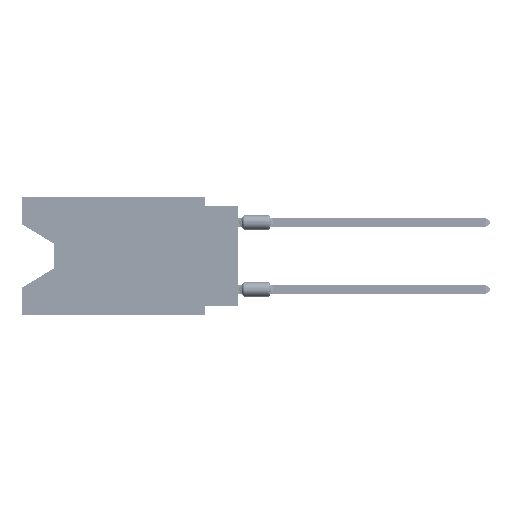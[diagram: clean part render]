
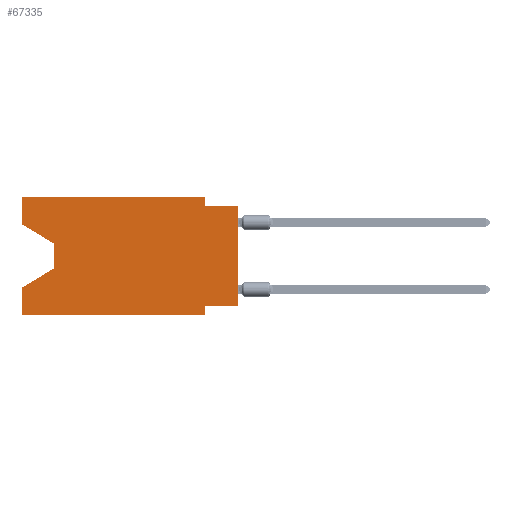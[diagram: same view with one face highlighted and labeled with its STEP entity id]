
A CAD part, left-side view. The second image highlights one B-rep face of the part: STEP entity #67335.
In plain terms, the highlighted planar face has unit normal (-1, 0, 0).
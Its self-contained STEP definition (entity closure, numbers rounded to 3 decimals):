
#154 = VERTEX_POINT ( 'NONE', #52740 ) ;
#1764 = EDGE_CURVE ( 'NONE', #3936, #50793, #80756, .T. ) ;
#3936 = VERTEX_POINT ( 'NONE', #56973 ) ;
#4220 = ORIENTED_EDGE ( 'NONE', *, *, #75615, .F. ) ;
#5803 = VECTOR ( 'NONE', #24884, 1000. ) ;
#6697 = PLANE ( 'NONE',  #82722 ) ;
#6852 = DIRECTION ( 'NONE',  ( 0., 0., -1. ) ) ;
#13258 = FACE_OUTER_BOUND ( 'NONE', #33063, .T. ) ;
#13718 = CARTESIAN_POINT ( 'NONE',  ( 0., 2.54, 0. ) ) ;
#14518 = DIRECTION ( 'NONE',  ( 0., 0., -1. ) ) ;
#15775 = DIRECTION ( 'NONE',  ( 0., -0.855, -0.519 ) ) ;
#16699 = CARTESIAN_POINT ( 'NONE',  ( 0., 16.383, 0. ) ) ;
#16708 = CARTESIAN_POINT ( 'NONE',  ( 0., 13.97, -5.385 ) ) ;
#16961 = ORIENTED_EDGE ( 'NONE', *, *, #58925, .F. ) ;
#18327 = LINE ( 'NONE', #37089, #5803 ) ;
#19431 = ORIENTED_EDGE ( 'NONE', *, *, #78847, .F. ) ;
#19486 = DIRECTION ( 'NONE',  ( 0., 0., 1. ) ) ;
#20074 = LINE ( 'NONE', #40119, #56451 ) ;
#20825 = CARTESIAN_POINT ( 'NONE',  ( 0., 16.383, 0. ) ) ;
#21880 = CARTESIAN_POINT ( 'NONE',  ( 0., 2.54, -8.89 ) ) ;
#22563 = CARTESIAN_POINT ( 'NONE',  ( 0., 16.383, -8.89 ) ) ;
#24884 = DIRECTION ( 'NONE',  ( 0., -1., 0. ) ) ;
#25660 = LINE ( 'NONE', #60813, #53903 ) ;
#25840 = ORIENTED_EDGE ( 'NONE', *, *, #66268, .T. ) ;
#25892 = DIRECTION ( 'NONE',  ( 1., 0., 0. ) ) ;
#26313 = CARTESIAN_POINT ( 'NONE',  ( 0., 13.97, -5.385 ) ) ;
#26903 = CARTESIAN_POINT ( 'NONE',  ( 0., 2.54, -8.89 ) ) ;
#28161 = VECTOR ( 'NONE', #61619, 1000. ) ;
#28951 = EDGE_CURVE ( 'NONE', #36471, #42325, #25660, .T. ) ;
#30410 = VERTEX_POINT ( 'NONE', #20825 ) ;
#31606 = ORIENTED_EDGE ( 'NONE', *, *, #36580, .F. ) ;
#32282 = VECTOR ( 'NONE', #19486, 1000. ) ;
#33063 = EDGE_LOOP ( 'NONE', ( #63339, #25840, #78708, #40700, #44068, #47706, #19431, #65410, #16961, #49831, #4220, #31606 ) ) ;
#34111 = CARTESIAN_POINT ( 'NONE',  ( 0., 16.383, -2.038 ) ) ;
#35208 = CARTESIAN_POINT ( 'NONE',  ( 0., 13.97, -3.505 ) ) ;
#35828 = CARTESIAN_POINT ( 'NONE',  ( 0., 13.97, -3.505 ) ) ;
#36471 = VERTEX_POINT ( 'NONE', #13718 ) ;
#36580 = EDGE_CURVE ( 'NONE', #3936, #30410, #49405, .T. ) ;
#37089 = CARTESIAN_POINT ( 'NONE',  ( 0., 16.383, 0. ) ) ;
#38062 = EDGE_CURVE ( 'NONE', #58208, #72092, #84050, .T. ) ;
#40119 = CARTESIAN_POINT ( 'NONE',  ( 0., 16.383, -8.89 ) ) ;
#40700 = ORIENTED_EDGE ( 'NONE', *, *, #56957, .F. ) ;
#41118 = CARTESIAN_POINT ( 'NONE',  ( 0., 16.383, 0. ) ) ;
#42325 = VERTEX_POINT ( 'NONE', #73325 ) ;
#42730 = VERTEX_POINT ( 'NONE', #44477 ) ;
#44068 = ORIENTED_EDGE ( 'NONE', *, *, #79811, .T. ) ;
#44477 = CARTESIAN_POINT ( 'NONE',  ( 0., 2.54, -8.255 ) ) ;
#45420 = LINE ( 'NONE', #52822, #58438 ) ;
#47706 = ORIENTED_EDGE ( 'NONE', *, *, #75015, .F. ) ;
#48466 = VECTOR ( 'NONE', #61262, 1000. ) ;
#49405 = LINE ( 'NONE', #16699, #28161 ) ;
#49831 = ORIENTED_EDGE ( 'NONE', *, *, #28951, .F. ) ;
#50088 = CARTESIAN_POINT ( 'NONE',  ( 0., 0., -8.255 ) ) ;
#50742 = VECTOR ( 'NONE', #77541, 1000. ) ;
#50793 = VERTEX_POINT ( 'NONE', #35208 ) ;
#51909 = VECTOR ( 'NONE', #15775, 1000. ) ;
#52740 = CARTESIAN_POINT ( 'NONE',  ( 0., 16.383, -6.852 ) ) ;
#52822 = CARTESIAN_POINT ( 'NONE',  ( 0., 0., -0.635 ) ) ;
#53903 = VECTOR ( 'NONE', #73477, 1000. ) ;
#56451 = VECTOR ( 'NONE', #68000, 1000. ) ;
#56808 = DIRECTION ( 'NONE',  ( 0., 0.855, -0.519 ) ) ;
#56957 = EDGE_CURVE ( 'NONE', #85426, #154, #67376, .T. ) ;
#56973 = CARTESIAN_POINT ( 'NONE',  ( 0., 16.383, -2.038 ) ) ;
#58208 = VERTEX_POINT ( 'NONE', #82607 ) ;
#58438 = VECTOR ( 'NONE', #85530, 1000. ) ;
#58925 = EDGE_CURVE ( 'NONE', #42325, #72092, #45420, .T. ) ;
#59196 = LINE ( 'NONE', #26903, #83839 ) ;
#60813 = CARTESIAN_POINT ( 'NONE',  ( 0., 2.54, 0. ) ) ;
#61262 = DIRECTION ( 'NONE',  ( 0., 0., 1. ) ) ;
#61619 = DIRECTION ( 'NONE',  ( 0., 0., 1. ) ) ;
#61695 = VECTOR ( 'NONE', #14518, 1000. ) ;
#63339 = ORIENTED_EDGE ( 'NONE', *, *, #1764, .T. ) ;
#64449 = LINE ( 'NONE', #50088, #50742 ) ;
#65410 = ORIENTED_EDGE ( 'NONE', *, *, #38062, .T. ) ;
#66268 = EDGE_CURVE ( 'NONE', #50793, #67395, #74235, .T. ) ;
#67335 = ADVANCED_FACE ( 'NONE', ( #13258 ), #6697, .F. ) ;
#67376 = LINE ( 'NONE', #74770, #48466 ) ;
#67395 = VERTEX_POINT ( 'NONE', #26313 ) ;
#68000 = DIRECTION ( 'NONE',  ( 0., -1., 0. ) ) ;
#72092 = VERTEX_POINT ( 'NONE', #79955 ) ;
#73325 = CARTESIAN_POINT ( 'NONE',  ( 0., 2.54, -0.635 ) ) ;
#73477 = DIRECTION ( 'NONE',  ( 0., 0., -1. ) ) ;
#74062 = VECTOR ( 'NONE', #56808, 1000. ) ;
#74225 = VERTEX_POINT ( 'NONE', #21880 ) ;
#74235 = LINE ( 'NONE', #35828, #61695 ) ;
#74770 = CARTESIAN_POINT ( 'NONE',  ( 0., 16.383, 0. ) ) ;
#75015 = EDGE_CURVE ( 'NONE', #42730, #74225, #59196, .T. ) ;
#75615 = EDGE_CURVE ( 'NONE', #30410, #36471, #18327, .T. ) ;
#76134 = EDGE_CURVE ( 'NONE', #67395, #154, #76425, .T. ) ;
#76425 = LINE ( 'NONE', #16708, #74062 ) ;
#77541 = DIRECTION ( 'NONE',  ( 0., 1., 0. ) ) ;
#78708 = ORIENTED_EDGE ( 'NONE', *, *, #76134, .T. ) ;
#78847 = EDGE_CURVE ( 'NONE', #58208, #42730, #64449, .T. ) ;
#79505 = DIRECTION ( 'NONE',  ( 0., 0., -1. ) ) ;
#79811 = EDGE_CURVE ( 'NONE', #85426, #74225, #20074, .T. ) ;
#79955 = CARTESIAN_POINT ( 'NONE',  ( 0., 0., -0.635 ) ) ;
#80756 = LINE ( 'NONE', #34111, #51909 ) ;
#82607 = CARTESIAN_POINT ( 'NONE',  ( 0., 0., -8.255 ) ) ;
#82722 = AXIS2_PLACEMENT_3D ( 'NONE', #41118, #25892, #79505 ) ;
#83839 = VECTOR ( 'NONE', #6852, 1000. ) ;
#84050 = LINE ( 'NONE', #84899, #32282 ) ;
#84899 = CARTESIAN_POINT ( 'NONE',  ( 0., 0., 0. ) ) ;
#85426 = VERTEX_POINT ( 'NONE', #22563 ) ;
#85530 = DIRECTION ( 'NONE',  ( 0., -1., 0. ) ) ;
